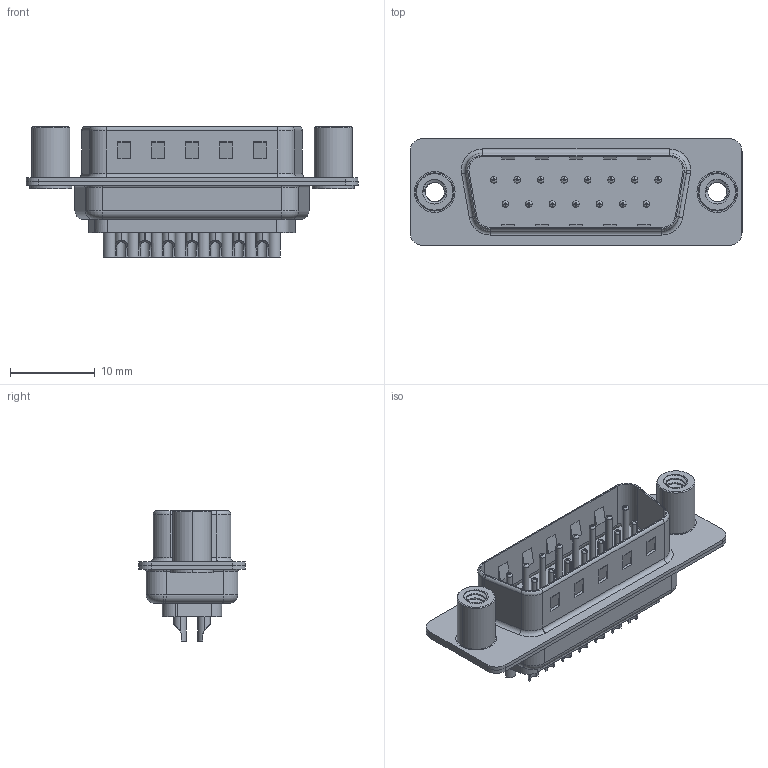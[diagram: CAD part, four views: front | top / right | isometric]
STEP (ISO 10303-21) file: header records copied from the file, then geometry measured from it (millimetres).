
FILE_DESCRIPTION (( 'STEP AP203' ), '1' );
FILE_NAME ('627-015-222-548.STEP', '2018-10-04T22:48:03', ( '' ), ( '' ), 'SwSTEP 2.0', 'SolidWorks 2016', '' );
FILE_SCHEMA (( 'CONFIG_CONTROL_DESIGN' ));
Length unit declared in the file: millimetre
Products named in the file (7): 627 Shell Front_15 Contacts; 627 Shell Rear_15 Contacts; 627 Contact Row 1_22L; 627 Contact Row 2_22L; 627 4-40 Threaded Standoff; 627-015-222-548; 627 Housing_15 LP
Assembly tree (20 placements, depth 2):
  627-015-222-548
    627 Housing_15 LP
    627 Shell Front_15 Contacts
    627 Shell Rear_15 Contacts
    627 Contact Row 1_22L  x8
    627 Contact Row 2_22L  x7
    627 4-40 Threaded Standoff  x2
Bounding box: 39.15 x 12.6 x 15.35 mm (x, y, z)
Volume: 1899.8 mm3; surface area: 5622.9 mm2
Topology: 20 solids, 20 shells, 1334 faces, 3411 edges, 2160 vertices
Faces by surface type: cylinder 596, torus 371, plane 351, cone 10, bspline 6
Entity records: 19642 total; most frequent: CARTESIAN_POINT 4779, DIRECTION 3077, ORIENTED_EDGE 2770, EDGE_CURVE 1385, AXIS2_PLACEMENT_3D 1213, VERTEX_POINT 881, EDGE_LOOP 660, VECTOR 651
